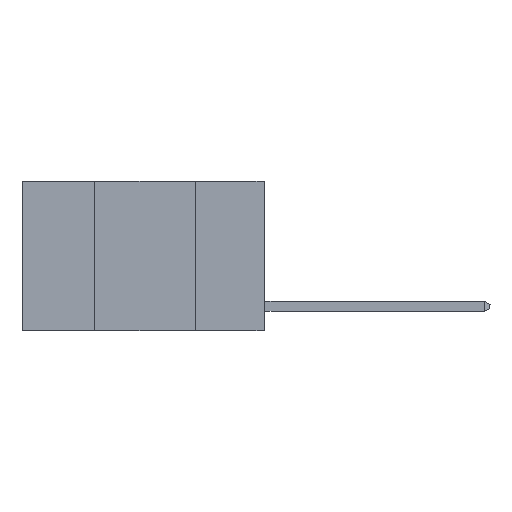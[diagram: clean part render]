
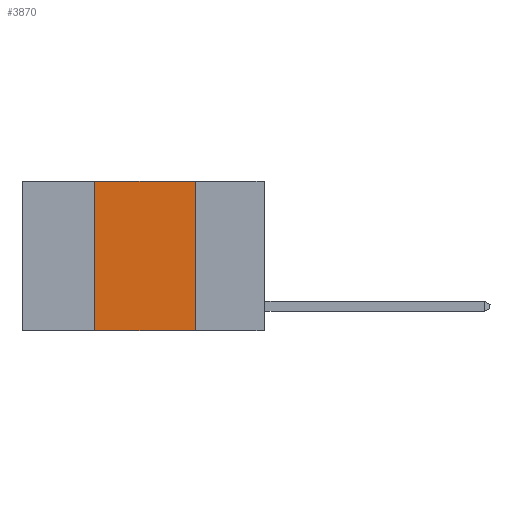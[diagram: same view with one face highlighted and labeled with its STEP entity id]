
A CAD part, left-side view. The second image highlights one B-rep face of the part: STEP entity #3870.
In plain terms, the highlighted planar face has unit normal (-1, 0, 0).
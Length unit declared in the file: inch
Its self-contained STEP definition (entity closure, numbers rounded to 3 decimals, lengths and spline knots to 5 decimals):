
#1397 = PLANE ( 'NONE',  #12103 ) ;
#2484 = LINE ( 'NONE', #15598, #9513 ) ;
#3870 = ADVANCED_FACE ( 'NONE', ( #16312 ), #1397, .F. ) ;
#4721 = VERTEX_POINT ( 'NONE', #7920 ) ;
#4851 = EDGE_CURVE ( 'NONE', #24155, #14410, #2484, .T. ) ;
#4925 = EDGE_CURVE ( 'NONE', #4721, #24155, #13384, .T. ) ;
#6808 = DIRECTION ( 'NONE',  ( 0., -1., 0. ) ) ;
#7920 = CARTESIAN_POINT ( 'NONE',  ( 0., 0.42, -0.37 ) ) ;
#8955 = CARTESIAN_POINT ( 'NONE',  ( 0., 0.6, 0. ) ) ;
#9513 = VECTOR ( 'NONE', #6808, 39.37008 ) ;
#10633 = VECTOR ( 'NONE', #22397, 39.37008 ) ;
#11881 = CARTESIAN_POINT ( 'NONE',  ( 0., 0.17, 0. ) ) ;
#12103 = AXIS2_PLACEMENT_3D ( 'NONE', #8955, #20513, #17484 ) ;
#13242 = VECTOR ( 'NONE', #22194, 39.37008 ) ;
#13384 = LINE ( 'NONE', #21898, #25165 ) ;
#13419 = VERTEX_POINT ( 'NONE', #20069 ) ;
#13692 = CARTESIAN_POINT ( 'NONE',  ( 0., 0.6, -0.37 ) ) ;
#14410 = VERTEX_POINT ( 'NONE', #11881 ) ;
#15553 = CARTESIAN_POINT ( 'NONE',  ( 0., 0.17, 0. ) ) ;
#15598 = CARTESIAN_POINT ( 'NONE',  ( 0., 0.6, 0. ) ) ;
#15771 = LINE ( 'NONE', #13692, #13242 ) ;
#16206 = EDGE_CURVE ( 'NONE', #4721, #13419, #15771, .T. ) ;
#16312 = FACE_OUTER_BOUND ( 'NONE', #20274, .T. ) ;
#17484 = DIRECTION ( 'NONE',  ( 0., 0., -1. ) ) ;
#18653 = EDGE_CURVE ( 'NONE', #14410, #13419, #20168, .T. ) ;
#18804 = ORIENTED_EDGE ( 'NONE', *, *, #16206, .T. ) ;
#20069 = CARTESIAN_POINT ( 'NONE',  ( 0., 0.17, -0.37 ) ) ;
#20168 = LINE ( 'NONE', #15553, #10633 ) ;
#20274 = EDGE_LOOP ( 'NONE', ( #21431, #21973, #22232, #18804 ) ) ;
#20513 = DIRECTION ( 'NONE',  ( 1., 0., 0. ) ) ;
#21431 = ORIENTED_EDGE ( 'NONE', *, *, #18653, .F. ) ;
#21873 = CARTESIAN_POINT ( 'NONE',  ( 0., 0.42, 0. ) ) ;
#21898 = CARTESIAN_POINT ( 'NONE',  ( 0., 0.42, 0. ) ) ;
#21973 = ORIENTED_EDGE ( 'NONE', *, *, #4851, .F. ) ;
#22194 = DIRECTION ( 'NONE',  ( 0., -1., 0. ) ) ;
#22232 = ORIENTED_EDGE ( 'NONE', *, *, #4925, .F. ) ;
#22397 = DIRECTION ( 'NONE',  ( 0., 0., -1. ) ) ;
#23591 = DIRECTION ( 'NONE',  ( 0., 0., 1. ) ) ;
#24155 = VERTEX_POINT ( 'NONE', #21873 ) ;
#25165 = VECTOR ( 'NONE', #23591, 39.37008 ) ;
